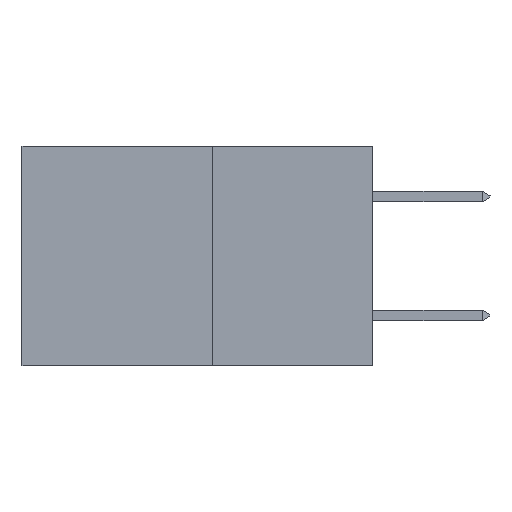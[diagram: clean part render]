
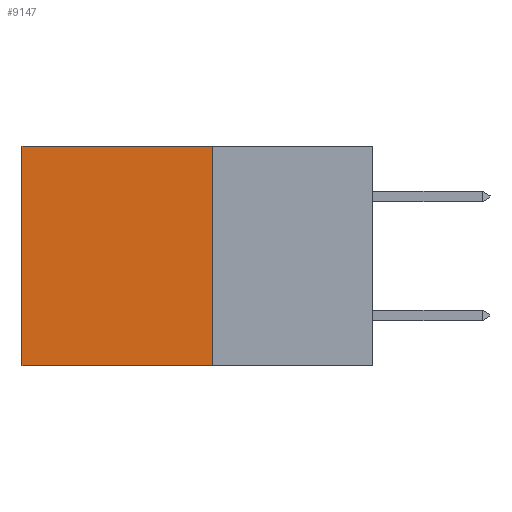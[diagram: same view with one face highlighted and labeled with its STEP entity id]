
A CAD part, left-side view. The second image highlights one B-rep face of the part: STEP entity #9147.
In plain terms, the highlighted planar face has unit normal (-1, 0, 0).
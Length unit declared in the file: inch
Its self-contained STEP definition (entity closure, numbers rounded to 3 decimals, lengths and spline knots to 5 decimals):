
#915 = CARTESIAN_POINT ( 'NONE',  ( 0.277, 0.27, 0. ) ) ;
#1450 = DIRECTION ( 'NONE',  ( 0., 0., -1. ) ) ;
#1593 = VECTOR ( 'NONE', #4876, 39.37008 ) ;
#3390 = ORIENTED_EDGE ( 'NONE', *, *, #24293, .F. ) ;
#4876 = DIRECTION ( 'NONE',  ( 0., 1., 0. ) ) ;
#5116 = ORIENTED_EDGE ( 'NONE', *, *, #21038, .T. ) ;
#5568 = CARTESIAN_POINT ( 'NONE',  ( 0.277, 0.27, -0.37 ) ) ;
#5839 = CARTESIAN_POINT ( 'NONE',  ( 0.277, 0.27, -0.37 ) ) ;
#6292 = CARTESIAN_POINT ( 'NONE',  ( 0.277, 0.59, -0.37 ) ) ;
#6585 = ORIENTED_EDGE ( 'NONE', *, *, #12799, .T. ) ;
#7215 = CARTESIAN_POINT ( 'NONE',  ( 0.277, 0.27, -0.37 ) ) ;
#8965 = FACE_OUTER_BOUND ( 'NONE', #15743, .T. ) ;
#9147 = ADVANCED_FACE ( 'NONE', ( #8965 ), #11227, .F. ) ;
#10321 = LINE ( 'NONE', #7215, #14165 ) ;
#11227 = PLANE ( 'NONE',  #15800 ) ;
#11306 = DIRECTION ( 'NONE',  ( 0., 0., -1. ) ) ;
#11315 = CARTESIAN_POINT ( 'NONE',  ( 0.277, 0.59, 0. ) ) ;
#11392 = CARTESIAN_POINT ( 'NONE',  ( 0.277, 0.27, 0. ) ) ;
#11558 = LINE ( 'NONE', #5839, #16465 ) ;
#11700 = DIRECTION ( 'NONE',  ( 0., 1., 0. ) ) ;
#12585 = ORIENTED_EDGE ( 'NONE', *, *, #23808, .F. ) ;
#12799 = EDGE_CURVE ( 'NONE', #14658, #16514, #22133, .T. ) ;
#12974 = VECTOR ( 'NONE', #11306, 39.37008 ) ;
#13126 = DIRECTION ( 'NONE',  ( 1., 0., 0. ) ) ;
#14165 = VECTOR ( 'NONE', #18543, 39.37008 ) ;
#14658 = VERTEX_POINT ( 'NONE', #11315 ) ;
#15743 = EDGE_LOOP ( 'NONE', ( #6585, #12585, #3390, #5116 ) ) ;
#15800 = AXIS2_PLACEMENT_3D ( 'NONE', #22237, #13126, #1450 ) ;
#16292 = VERTEX_POINT ( 'NONE', #11392 ) ;
#16319 = LINE ( 'NONE', #915, #1593 ) ;
#16465 = VECTOR ( 'NONE', #11700, 39.37008 ) ;
#16514 = VERTEX_POINT ( 'NONE', #6292 ) ;
#16909 = VERTEX_POINT ( 'NONE', #5568 ) ;
#18543 = DIRECTION ( 'NONE',  ( 0., 0., -1. ) ) ;
#21038 = EDGE_CURVE ( 'NONE', #16292, #14658, #16319, .T. ) ;
#22133 = LINE ( 'NONE', #24202, #12974 ) ;
#22237 = CARTESIAN_POINT ( 'NONE',  ( 0.277, 0.27, -0.37 ) ) ;
#23808 = EDGE_CURVE ( 'NONE', #16909, #16514, #11558, .T. ) ;
#24202 = CARTESIAN_POINT ( 'NONE',  ( 0.277, 0.59, -0.37 ) ) ;
#24293 = EDGE_CURVE ( 'NONE', #16292, #16909, #10321, .T. ) ;
